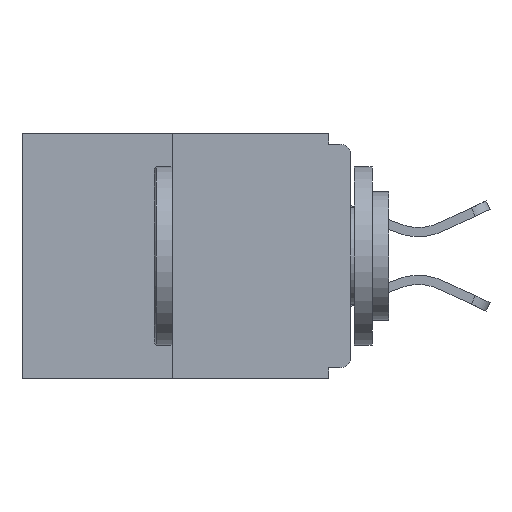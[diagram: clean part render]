
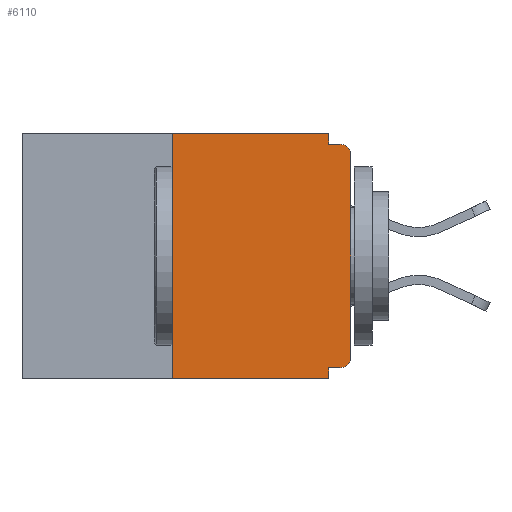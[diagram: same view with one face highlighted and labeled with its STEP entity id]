
A CAD part, left-side view. The second image highlights one B-rep face of the part: STEP entity #6110.
In plain terms, the highlighted planar face has unit normal (-1, 0, 0).
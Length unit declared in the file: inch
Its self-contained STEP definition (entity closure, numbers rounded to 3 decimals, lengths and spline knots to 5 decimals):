
#44 = CIRCLE ( 'NONE', #7892, 0.015 ) ;
#281 = PLANE ( 'NONE',  #5153 ) ;
#405 = DIRECTION ( 'NONE',  ( 0., 0., -1. ) ) ;
#696 = DIRECTION ( 'NONE',  ( 0., -1., 0. ) ) ;
#1003 = EDGE_CURVE ( 'NONE', #5938, #15663, #3617, .T. ) ;
#1127 = EDGE_CURVE ( 'NONE', #10806, #15663, #5408, .T. ) ;
#1683 = CARTESIAN_POINT ( 'NONE',  ( 0., 0.46, 0. ) ) ;
#1931 = CARTESIAN_POINT ( 'NONE',  ( 0., 0.015, -0.015 ) ) ;
#2001 = ORIENTED_EDGE ( 'NONE', *, *, #17328, .F. ) ;
#2637 = ORIENTED_EDGE ( 'NONE', *, *, #16104, .F. ) ;
#2777 = EDGE_CURVE ( 'NONE', #6844, #2870, #44, .T. ) ;
#2870 = VERTEX_POINT ( 'NONE', #15886 ) ;
#3081 = VERTEX_POINT ( 'NONE', #17426 ) ;
#3095 = CARTESIAN_POINT ( 'NONE',  ( 0., 0.031, -0.343 ) ) ;
#3192 = DIRECTION ( 'NONE',  ( 0., -1., 0. ) ) ;
#3197 = DIRECTION ( 'NONE',  ( 1., 0., 0. ) ) ;
#3323 = LINE ( 'NONE', #17778, #8764 ) ;
#3394 = ORIENTED_EDGE ( 'NONE', *, *, #2777, .T. ) ;
#3577 = CARTESIAN_POINT ( 'NONE',  ( 0., 0.46, -0.343 ) ) ;
#3590 = CARTESIAN_POINT ( 'NONE',  ( 0., 0., -0.015 ) ) ;
#3617 = LINE ( 'NONE', #3095, #18681 ) ;
#3745 = CARTESIAN_POINT ( 'NONE',  ( 0., 0.031, -0.015 ) ) ;
#4260 = CARTESIAN_POINT ( 'NONE',  ( 0., 0., 0. ) ) ;
#4979 = DIRECTION ( 'NONE',  ( 0., 1., 0. ) ) ;
#5141 = LINE ( 'NONE', #16629, #17273 ) ;
#5153 = AXIS2_PLACEMENT_3D ( 'NONE', #1683, #3197, #405 ) ;
#5214 = CARTESIAN_POINT ( 'NONE',  ( 0., 0.015, -0.03 ) ) ;
#5351 = DIRECTION ( 'NONE',  ( -1., 0., 0. ) ) ;
#5408 = LINE ( 'NONE', #3577, #15244 ) ;
#5938 = VERTEX_POINT ( 'NONE', #11923 ) ;
#6110 = ADVANCED_FACE ( 'NONE', ( #18201 ), #281, .F. ) ;
#6282 = VERTEX_POINT ( 'NONE', #3745 ) ;
#6300 = ORIENTED_EDGE ( 'NONE', *, *, #12636, .F. ) ;
#6844 = VERTEX_POINT ( 'NONE', #11041 ) ;
#6871 = EDGE_CURVE ( 'NONE', #11935, #14884, #9676, .T. ) ;
#7087 = CARTESIAN_POINT ( 'NONE',  ( 0., 0.031, 0. ) ) ;
#7788 = ORIENTED_EDGE ( 'NONE', *, *, #6871, .T. ) ;
#7892 = AXIS2_PLACEMENT_3D ( 'NONE', #12644, #5351, #15567 ) ;
#8534 = DIRECTION ( 'NONE',  ( 0., 0., 1. ) ) ;
#8568 = ORIENTED_EDGE ( 'NONE', *, *, #18018, .F. ) ;
#8764 = VECTOR ( 'NONE', #3192, 39.37008 ) ;
#9172 = DIRECTION ( 'NONE',  ( 0., -1., 0. ) ) ;
#9676 = CIRCLE ( 'NONE', #10296, 0.015 ) ;
#10296 = AXIS2_PLACEMENT_3D ( 'NONE', #5214, #15438, #18454 ) ;
#10549 = CARTESIAN_POINT ( 'NONE',  ( 0., 0.25, -0.343 ) ) ;
#10743 = LINE ( 'NONE', #18712, #11195 ) ;
#10806 = VERTEX_POINT ( 'NONE', #10549 ) ;
#10820 = ORIENTED_EDGE ( 'NONE', *, *, #11475, .T. ) ;
#10914 = ORIENTED_EDGE ( 'NONE', *, *, #13590, .F. ) ;
#10978 = VECTOR ( 'NONE', #14403, 39.37008 ) ;
#11033 = VECTOR ( 'NONE', #16164, 39.37008 ) ;
#11041 = CARTESIAN_POINT ( 'NONE',  ( 0., 0.015, -0.328 ) ) ;
#11195 = VECTOR ( 'NONE', #8534, 39.37008 ) ;
#11475 = EDGE_CURVE ( 'NONE', #2870, #11935, #15376, .T. ) ;
#11881 = LINE ( 'NONE', #7087, #10978 ) ;
#11923 = CARTESIAN_POINT ( 'NONE',  ( 0., 0.031, -0.328 ) ) ;
#11935 = VERTEX_POINT ( 'NONE', #12359 ) ;
#12359 = CARTESIAN_POINT ( 'NONE',  ( 0., 0., -0.03 ) ) ;
#12485 = VERTEX_POINT ( 'NONE', #12745 ) ;
#12636 = EDGE_CURVE ( 'NONE', #3081, #6282, #11881, .T. ) ;
#12644 = CARTESIAN_POINT ( 'NONE',  ( 0., 0.015, -0.313 ) ) ;
#12745 = CARTESIAN_POINT ( 'NONE',  ( 0., 0.25, 0. ) ) ;
#13185 = VECTOR ( 'NONE', #9172, 39.37008 ) ;
#13590 = EDGE_CURVE ( 'NONE', #10806, #12485, #10743, .T. ) ;
#13646 = ORIENTED_EDGE ( 'NONE', *, *, #1127, .T. ) ;
#14403 = DIRECTION ( 'NONE',  ( 0., 0., -1. ) ) ;
#14468 = DIRECTION ( 'NONE',  ( 0., 0., -1. ) ) ;
#14884 = VERTEX_POINT ( 'NONE', #1931 ) ;
#15244 = VECTOR ( 'NONE', #696, 39.37008 ) ;
#15376 = LINE ( 'NONE', #4260, #11033 ) ;
#15438 = DIRECTION ( 'NONE',  ( -1., 0., 0. ) ) ;
#15567 = DIRECTION ( 'NONE',  ( 0., 0., -1. ) ) ;
#15639 = ORIENTED_EDGE ( 'NONE', *, *, #1003, .F. ) ;
#15663 = VERTEX_POINT ( 'NONE', #18017 ) ;
#15886 = CARTESIAN_POINT ( 'NONE',  ( 0., 0., -0.313 ) ) ;
#16104 = EDGE_CURVE ( 'NONE', #6282, #14884, #18012, .T. ) ;
#16164 = DIRECTION ( 'NONE',  ( 0., 0., 1. ) ) ;
#16629 = CARTESIAN_POINT ( 'NONE',  ( 0., 0., -0.328 ) ) ;
#17273 = VECTOR ( 'NONE', #4979, 39.37008 ) ;
#17328 = EDGE_CURVE ( 'NONE', #6844, #5938, #5141, .T. ) ;
#17426 = CARTESIAN_POINT ( 'NONE',  ( 0., 0.031, 0. ) ) ;
#17778 = CARTESIAN_POINT ( 'NONE',  ( 0., 0.46, 0. ) ) ;
#17981 = EDGE_LOOP ( 'NONE', ( #8568, #10914, #13646, #15639, #2001, #3394, #10820, #7788, #2637, #6300 ) ) ;
#18012 = LINE ( 'NONE', #3590, #13185 ) ;
#18017 = CARTESIAN_POINT ( 'NONE',  ( 0., 0.031, -0.343 ) ) ;
#18018 = EDGE_CURVE ( 'NONE', #12485, #3081, #3323, .T. ) ;
#18201 = FACE_OUTER_BOUND ( 'NONE', #17981, .T. ) ;
#18454 = DIRECTION ( 'NONE',  ( 0., 0., -1. ) ) ;
#18681 = VECTOR ( 'NONE', #14468, 39.37008 ) ;
#18712 = CARTESIAN_POINT ( 'NONE',  ( 0., 0.25, 0. ) ) ;
